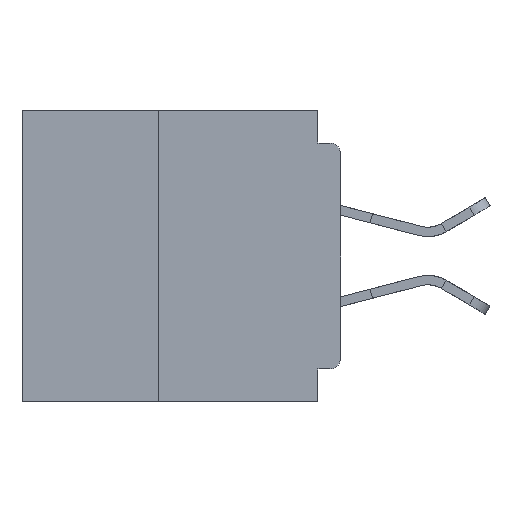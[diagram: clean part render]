
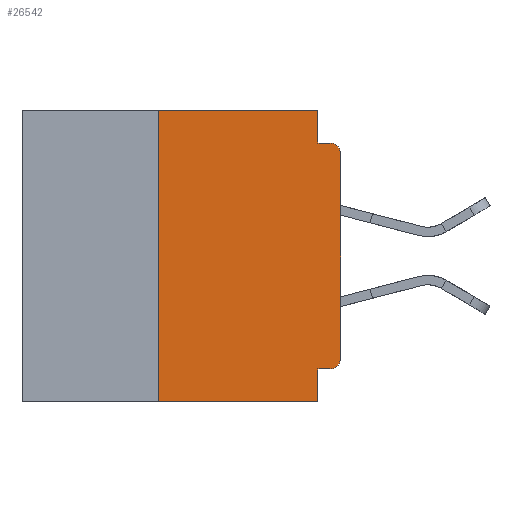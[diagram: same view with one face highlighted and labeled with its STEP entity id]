
A CAD part, left-side view. The second image highlights one B-rep face of the part: STEP entity #26542.
In plain terms, the highlighted planar face has unit normal (-1, 0, 0).
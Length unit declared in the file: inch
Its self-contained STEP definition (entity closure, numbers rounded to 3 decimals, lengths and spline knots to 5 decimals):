
#6 = DIRECTION ( 'NONE',  ( -1., 0., 0. ) ) ;
#638 = EDGE_CURVE ( 'NONE', #8577, #28783, #10625, .T. ) ;
#878 = DIRECTION ( 'NONE',  ( 0., -1., 0. ) ) ;
#1268 = CARTESIAN_POINT ( 'NONE',  ( 0., 0.031, 0. ) ) ;
#2318 = EDGE_LOOP ( 'NONE', ( #29265, #10794, #38046, #28118, #29149, #20833, #14516, #23424, #15594, #5780 ) ) ;
#2586 = DIRECTION ( 'NONE',  ( 1., 0., 0. ) ) ;
#2832 = LINE ( 'NONE', #18104, #19033 ) ;
#3055 = LINE ( 'NONE', #39458, #27817 ) ;
#3922 = EDGE_CURVE ( 'NONE', #19782, #4521, #7908, .T. ) ;
#4521 = VERTEX_POINT ( 'NONE', #25007 ) ;
#5780 = ORIENTED_EDGE ( 'NONE', *, *, #31699, .T. ) ;
#6407 = EDGE_CURVE ( 'NONE', #37209, #8577, #2832, .T. ) ;
#7008 = CARTESIAN_POINT ( 'NONE',  ( 0., 0.031, -0.355 ) ) ;
#7540 = VERTEX_POINT ( 'NONE', #12532 ) ;
#7908 = LINE ( 'NONE', #12956, #23076 ) ;
#8577 = VERTEX_POINT ( 'NONE', #21673 ) ;
#9181 = VECTOR ( 'NONE', #29103, 39.37008 ) ;
#9205 = VECTOR ( 'NONE', #9507, 39.37008 ) ;
#9357 = EDGE_CURVE ( 'NONE', #7540, #19782, #35864, .T. ) ;
#9455 = CARTESIAN_POINT ( 'NONE',  ( 0., 0.25, -0.4 ) ) ;
#9507 = DIRECTION ( 'NONE',  ( 0., -1., 0. ) ) ;
#10409 = EDGE_CURVE ( 'NONE', #29651, #4521, #3055, .T. ) ;
#10625 = CIRCLE ( 'NONE', #16335, 0.015 ) ;
#10794 = ORIENTED_EDGE ( 'NONE', *, *, #638, .T. ) ;
#12532 = CARTESIAN_POINT ( 'NONE',  ( 0., 0.015, -0.355 ) ) ;
#12562 = EDGE_CURVE ( 'NONE', #29651, #37364, #19047, .T. ) ;
#12956 = CARTESIAN_POINT ( 'NONE',  ( 0., 0.031, -0.4 ) ) ;
#13086 = LINE ( 'NONE', #24840, #20685 ) ;
#13611 = DIRECTION ( 'NONE',  ( -1., 0., 0. ) ) ;
#14516 = ORIENTED_EDGE ( 'NONE', *, *, #10409, .T. ) ;
#15512 = CARTESIAN_POINT ( 'NONE',  ( 0., 0.015, -0.06 ) ) ;
#15594 = ORIENTED_EDGE ( 'NONE', *, *, #9357, .F. ) ;
#15842 = CARTESIAN_POINT ( 'NONE',  ( 0., 0.437, 0. ) ) ;
#16181 = DIRECTION ( 'NONE',  ( 0., 0., -1. ) ) ;
#16335 = AXIS2_PLACEMENT_3D ( 'NONE', #15512, #13611, #18832 ) ;
#16918 = EDGE_CURVE ( 'NONE', #36512, #25108, #13086, .T. ) ;
#18010 = CARTESIAN_POINT ( 'NONE',  ( 0., 0.031, -0.045 ) ) ;
#18104 = CARTESIAN_POINT ( 'NONE',  ( 0., 0., 0. ) ) ;
#18832 = DIRECTION ( 'NONE',  ( 0., 0., -1. ) ) ;
#19033 = VECTOR ( 'NONE', #21333, 39.37008 ) ;
#19047 = LINE ( 'NONE', #21696, #35053 ) ;
#19449 = CARTESIAN_POINT ( 'NONE',  ( 0., 0.015, -0.34 ) ) ;
#19782 = VERTEX_POINT ( 'NONE', #7008 ) ;
#20685 = VECTOR ( 'NONE', #31102, 39.37008 ) ;
#20833 = ORIENTED_EDGE ( 'NONE', *, *, #12562, .F. ) ;
#21333 = DIRECTION ( 'NONE',  ( 0., 0., 1. ) ) ;
#21611 = CARTESIAN_POINT ( 'NONE',  ( 0., 0., -0.34 ) ) ;
#21646 = AXIS2_PLACEMENT_3D ( 'NONE', #21990, #2586, #25219 ) ;
#21673 = CARTESIAN_POINT ( 'NONE',  ( 0., 0., -0.06 ) ) ;
#21696 = CARTESIAN_POINT ( 'NONE',  ( 0., 0.25, -0.4 ) ) ;
#21990 = CARTESIAN_POINT ( 'NONE',  ( 0., 0.437, 0. ) ) ;
#22682 = CARTESIAN_POINT ( 'NONE',  ( 0., 0., -0.045 ) ) ;
#22715 = DIRECTION ( 'NONE',  ( 0., 0., -1. ) ) ;
#23076 = VECTOR ( 'NONE', #16181, 39.37008 ) ;
#23424 = ORIENTED_EDGE ( 'NONE', *, *, #3922, .F. ) ;
#24840 = CARTESIAN_POINT ( 'NONE',  ( 0., 0.031, 0. ) ) ;
#24872 = FACE_OUTER_BOUND ( 'NONE', #2318, .T. ) ;
#25007 = CARTESIAN_POINT ( 'NONE',  ( 0., 0.031, -0.4 ) ) ;
#25108 = VERTEX_POINT ( 'NONE', #18010 ) ;
#25219 = DIRECTION ( 'NONE',  ( 0., 0., -1. ) ) ;
#25280 = AXIS2_PLACEMENT_3D ( 'NONE', #19449, #6, #22715 ) ;
#26401 = LINE ( 'NONE', #15842, #9205 ) ;
#26542 = ADVANCED_FACE ( 'NONE', ( #24872 ), #41106, .F. ) ;
#26691 = EDGE_CURVE ( 'NONE', #25108, #28783, #34807, .T. ) ;
#27411 = VECTOR ( 'NONE', #38345, 39.37008 ) ;
#27817 = VECTOR ( 'NONE', #878, 39.37008 ) ;
#28118 = ORIENTED_EDGE ( 'NONE', *, *, #16918, .F. ) ;
#28153 = DIRECTION ( 'NONE',  ( 0., 0., 1. ) ) ;
#28783 = VERTEX_POINT ( 'NONE', #30638 ) ;
#28872 = CARTESIAN_POINT ( 'NONE',  ( 0., 0.25, 0. ) ) ;
#29103 = DIRECTION ( 'NONE',  ( 0., -1., 0. ) ) ;
#29149 = ORIENTED_EDGE ( 'NONE', *, *, #32299, .F. ) ;
#29265 = ORIENTED_EDGE ( 'NONE', *, *, #6407, .T. ) ;
#29651 = VERTEX_POINT ( 'NONE', #9455 ) ;
#30638 = CARTESIAN_POINT ( 'NONE',  ( 0., 0.015, -0.045 ) ) ;
#31102 = DIRECTION ( 'NONE',  ( 0., 0., -1. ) ) ;
#31699 = EDGE_CURVE ( 'NONE', #7540, #37209, #33413, .T. ) ;
#32299 = EDGE_CURVE ( 'NONE', #37364, #36512, #26401, .T. ) ;
#33413 = CIRCLE ( 'NONE', #25280, 0.015 ) ;
#34807 = LINE ( 'NONE', #22682, #9181 ) ;
#35053 = VECTOR ( 'NONE', #28153, 39.37008 ) ;
#35864 = LINE ( 'NONE', #38215, #27411 ) ;
#36512 = VERTEX_POINT ( 'NONE', #1268 ) ;
#37209 = VERTEX_POINT ( 'NONE', #21611 ) ;
#37364 = VERTEX_POINT ( 'NONE', #28872 ) ;
#38046 = ORIENTED_EDGE ( 'NONE', *, *, #26691, .F. ) ;
#38215 = CARTESIAN_POINT ( 'NONE',  ( 0., 0., -0.355 ) ) ;
#38345 = DIRECTION ( 'NONE',  ( 0., 1., 0. ) ) ;
#39458 = CARTESIAN_POINT ( 'NONE',  ( 0., 0.437, -0.4 ) ) ;
#41106 = PLANE ( 'NONE',  #21646 ) ;
